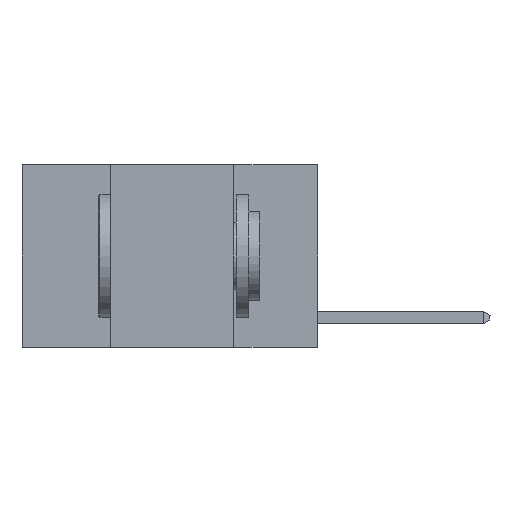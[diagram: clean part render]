
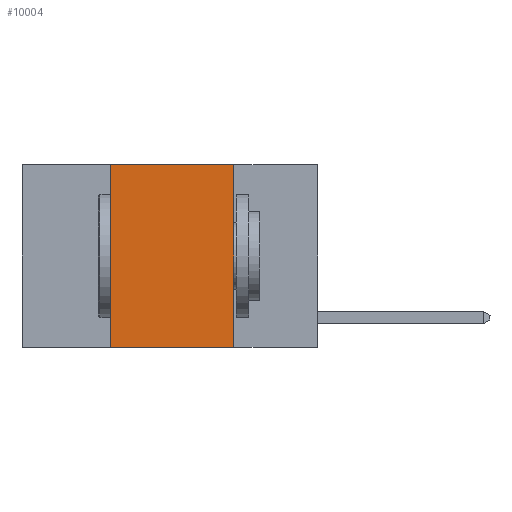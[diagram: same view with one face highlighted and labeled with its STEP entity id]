
A CAD part, left-side view. The second image highlights one B-rep face of the part: STEP entity #10004.
In plain terms, the highlighted planar face has unit normal (-1, 0, 0).
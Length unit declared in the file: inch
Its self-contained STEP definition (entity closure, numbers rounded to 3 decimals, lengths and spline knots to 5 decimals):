
#578 = EDGE_CURVE ( 'NONE', #3112, #13018, #1105, .T. ) ;
#947 = EDGE_CURVE ( 'NONE', #13018, #2399, #2732, .T. ) ;
#1105 = LINE ( 'NONE', #12315, #4057 ) ;
#1216 = PLANE ( 'NONE',  #3130 ) ;
#1402 = ORIENTED_EDGE ( 'NONE', *, *, #6836, .T. ) ;
#1831 = CARTESIAN_POINT ( 'NONE',  ( 0., 0.6, 0. ) ) ;
#2154 = DIRECTION ( 'NONE',  ( 0., 0., -1. ) ) ;
#2298 = CARTESIAN_POINT ( 'NONE',  ( 0., 0.42, -0.37 ) ) ;
#2399 = VERTEX_POINT ( 'NONE', #8192 ) ;
#2556 = LINE ( 'NONE', #10817, #7781 ) ;
#2668 = VECTOR ( 'NONE', #3908, 39.37008 ) ;
#2732 = LINE ( 'NONE', #1831, #2668 ) ;
#3112 = VERTEX_POINT ( 'NONE', #2298 ) ;
#3130 = AXIS2_PLACEMENT_3D ( 'NONE', #3322, #3249, #2154 ) ;
#3153 = LINE ( 'NONE', #4133, #10385 ) ;
#3249 = DIRECTION ( 'NONE',  ( 1., 0., 0. ) ) ;
#3322 = CARTESIAN_POINT ( 'NONE',  ( 0., 0.6, 0. ) ) ;
#3555 = EDGE_CURVE ( 'NONE', #2399, #7029, #3153, .T. ) ;
#3908 = DIRECTION ( 'NONE',  ( 0., -1., 0. ) ) ;
#4057 = VECTOR ( 'NONE', #12124, 39.37008 ) ;
#4067 = CARTESIAN_POINT ( 'NONE',  ( 0., 0.17, -0.37 ) ) ;
#4133 = CARTESIAN_POINT ( 'NONE',  ( 0., 0.17, 0. ) ) ;
#4145 = EDGE_LOOP ( 'NONE', ( #9600, #12472, #4179, #1402 ) ) ;
#4179 = ORIENTED_EDGE ( 'NONE', *, *, #578, .F. ) ;
#4730 = DIRECTION ( 'NONE',  ( 0., -1., 0. ) ) ;
#5354 = FACE_OUTER_BOUND ( 'NONE', #4145, .T. ) ;
#6836 = EDGE_CURVE ( 'NONE', #3112, #7029, #2556, .T. ) ;
#7029 = VERTEX_POINT ( 'NONE', #4067 ) ;
#7781 = VECTOR ( 'NONE', #4730, 39.37008 ) ;
#8192 = CARTESIAN_POINT ( 'NONE',  ( 0., 0.17, 0. ) ) ;
#9600 = ORIENTED_EDGE ( 'NONE', *, *, #3555, .F. ) ;
#9611 = CARTESIAN_POINT ( 'NONE',  ( 0., 0.42, 0. ) ) ;
#10004 = ADVANCED_FACE ( 'NONE', ( #5354 ), #1216, .F. ) ;
#10385 = VECTOR ( 'NONE', #11285, 39.37008 ) ;
#10817 = CARTESIAN_POINT ( 'NONE',  ( 0., 0.6, -0.37 ) ) ;
#11285 = DIRECTION ( 'NONE',  ( 0., 0., -1. ) ) ;
#12124 = DIRECTION ( 'NONE',  ( 0., 0., 1. ) ) ;
#12315 = CARTESIAN_POINT ( 'NONE',  ( 0., 0.42, 0. ) ) ;
#12472 = ORIENTED_EDGE ( 'NONE', *, *, #947, .F. ) ;
#13018 = VERTEX_POINT ( 'NONE', #9611 ) ;
